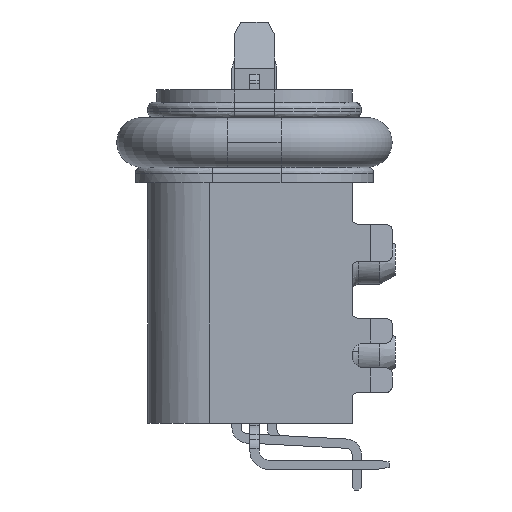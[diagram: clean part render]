
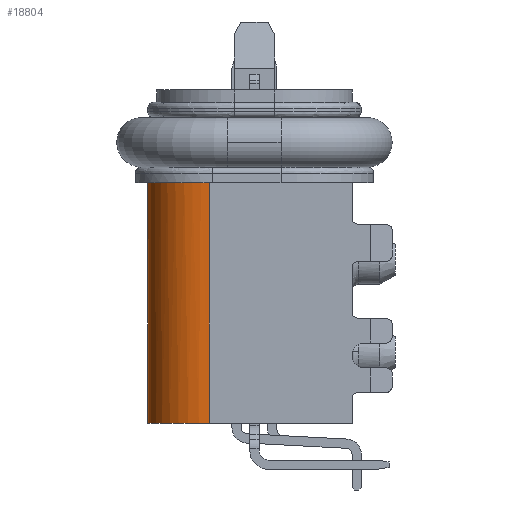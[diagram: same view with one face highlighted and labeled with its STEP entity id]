
A CAD part, left-side view. The second image highlights one B-rep face of the part: STEP entity #18804.
In plain terms, the highlighted cylindrical face has radius 1 mm (diameter 2 mm), a partial arc.
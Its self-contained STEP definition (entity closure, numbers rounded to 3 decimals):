
#157 = EDGE_CURVE ( 'NONE', #5643, #24958, #11622, .T. ) ;
#1666 = CARTESIAN_POINT ( 'NONE',  ( -3.795, 1.75, -2. ) ) ;
#2161 = DIRECTION ( 'NONE',  ( 0., 0., -1. ) ) ;
#3034 = AXIS2_PLACEMENT_3D ( 'NONE', #8027, #6278, #14374 ) ;
#3815 = ORIENTED_EDGE ( 'NONE', *, *, #22447, .F. ) ;
#4225 = CARTESIAN_POINT ( 'NONE',  ( -4.759, 1.027, 1.9 ) ) ;
#5643 = VERTEX_POINT ( 'NONE', #17105 ) ;
#6278 = DIRECTION ( 'NONE',  ( 0., 0., 1. ) ) ;
#6956 = DIRECTION ( 'NONE',  ( 1., 0., 0. ) ) ;
#7125 = CARTESIAN_POINT ( 'NONE',  ( -4.795, 0.75, -2. ) ) ;
#7374 = DIRECTION ( 'NONE',  ( 0., 0., 1. ) ) ;
#8027 = CARTESIAN_POINT ( 'NONE',  ( -3.795, 0.75, -9.039 ) ) ;
#8109 = ORIENTED_EDGE ( 'NONE', *, *, #157, .F. ) ;
#8176 = DIRECTION ( 'NONE',  ( 1., 0., 0. ) ) ;
#8552 = CIRCLE ( 'NONE', #18636, 1. ) ;
#8922 = ORIENTED_EDGE ( 'NONE', *, *, #18312, .T. ) ;
#9302 = VERTEX_POINT ( 'NONE', #11042 ) ;
#9869 = CYLINDRICAL_SURFACE ( 'NONE', #3034, 1. ) ;
#10372 = DIRECTION ( 'NONE',  ( 0., 0., 1. ) ) ;
#11042 = CARTESIAN_POINT ( 'NONE',  ( -3.795, 1.75, 1.9 ) ) ;
#11622 = B_SPLINE_CURVE_WITH_KNOTS ( 'NONE', 3,
 ( #20268, #4225, #12225, #16196 ),
 .UNSPECIFIED., .F., .F.,
 ( 4, 4 ),
 ( 0., 1. ),
 .UNSPECIFIED. ) ;
#11776 = LINE ( 'NONE', #21388, #15766 ) ;
#12085 = VERTEX_POINT ( 'NONE', #1666 ) ;
#12225 = CARTESIAN_POINT ( 'NONE',  ( -4.788, 0.889, 1.9 ) ) ;
#12611 = LINE ( 'NONE', #18307, #18347 ) ;
#13874 = ORIENTED_EDGE ( 'NONE', *, *, #22888, .T. ) ;
#14374 = DIRECTION ( 'NONE',  ( 1., 0., 0. ) ) ;
#15488 = CARTESIAN_POINT ( 'NONE',  ( -4.795, 0.75, 1.9 ) ) ;
#15766 = VECTOR ( 'NONE', #7374, 1000. ) ;
#15858 = VERTEX_POINT ( 'NONE', #7125 ) ;
#16196 = CARTESIAN_POINT ( 'NONE',  ( -4.795, 0.75, 1.9 ) ) ;
#16307 = EDGE_CURVE ( 'NONE', #5643, #9302, #8552, .T. ) ;
#17105 = CARTESIAN_POINT ( 'NONE',  ( -4.709, 1.156, 1.9 ) ) ;
#17163 = CARTESIAN_POINT ( 'NONE',  ( -3.795, 0.75, -2. ) ) ;
#18239 = CARTESIAN_POINT ( 'NONE',  ( -3.795, 0.75, 1.9 ) ) ;
#18307 = CARTESIAN_POINT ( 'NONE',  ( -3.795, 1.75, -0.3 ) ) ;
#18312 = EDGE_CURVE ( 'NONE', #15858, #24958, #11776, .T. ) ;
#18347 = VECTOR ( 'NONE', #10372, 1000. ) ;
#18636 = AXIS2_PLACEMENT_3D ( 'NONE', #18239, #2161, #8176 ) ;
#18804 = ADVANCED_FACE ( 'NONE', ( #24026 ), #9869, .T. ) ;
#19378 = DIRECTION ( 'NONE',  ( 0., 0., 1. ) ) ;
#19616 = CIRCLE ( 'NONE', #22563, 1. ) ;
#20268 = CARTESIAN_POINT ( 'NONE',  ( -4.709, 1.156, 1.9 ) ) ;
#21388 = CARTESIAN_POINT ( 'NONE',  ( -4.795, 0.75, -2. ) ) ;
#22447 = EDGE_CURVE ( 'NONE', #12085, #9302, #12611, .T. ) ;
#22563 = AXIS2_PLACEMENT_3D ( 'NONE', #17163, #19378, #6956 ) ;
#22624 = EDGE_LOOP ( 'NONE', ( #8922, #8109, #25489, #3815, #13874 ) ) ;
#22888 = EDGE_CURVE ( 'NONE', #12085, #15858, #19616, .T. ) ;
#24026 = FACE_OUTER_BOUND ( 'NONE', #22624, .T. ) ;
#24958 = VERTEX_POINT ( 'NONE', #15488 ) ;
#25489 = ORIENTED_EDGE ( 'NONE', *, *, #16307, .T. ) ;
